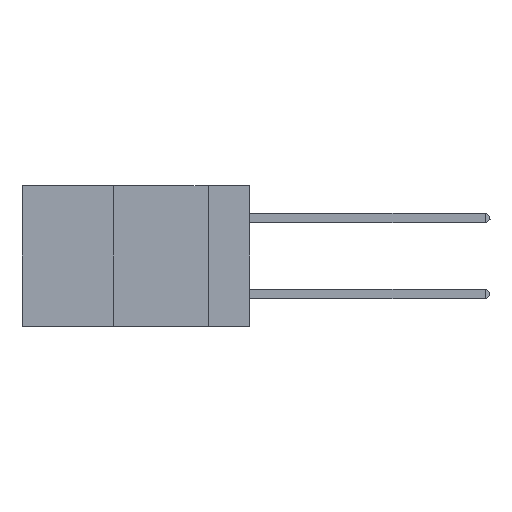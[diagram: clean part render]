
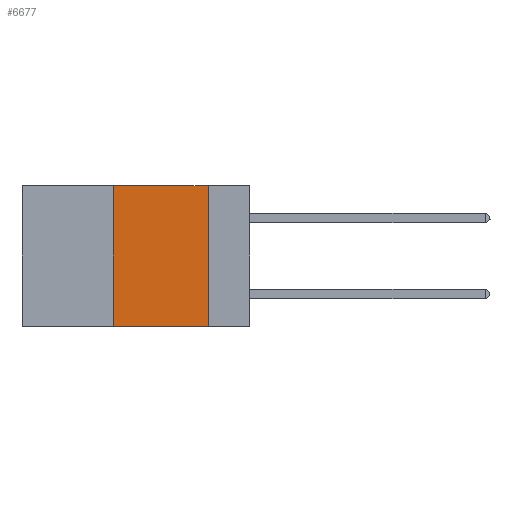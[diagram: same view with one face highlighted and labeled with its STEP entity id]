
A CAD part, left-side view. The second image highlights one B-rep face of the part: STEP entity #6677.
In plain terms, the highlighted planar face has unit normal (-1, 0, 0).
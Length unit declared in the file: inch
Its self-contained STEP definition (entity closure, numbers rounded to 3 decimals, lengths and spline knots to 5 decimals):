
#34 = LINE ( 'NONE', #2917, #3420 ) ;
#518 = DIRECTION ( 'NONE',  ( 0., 0., -1. ) ) ;
#813 = CARTESIAN_POINT ( 'NONE',  ( 0., 0.11, -0.37 ) ) ;
#999 = EDGE_CURVE ( 'NONE', #1155, #1673, #34, .T. ) ;
#1155 = VERTEX_POINT ( 'NONE', #3032 ) ;
#1369 = CARTESIAN_POINT ( 'NONE',  ( 0., 0.11, 0. ) ) ;
#1428 = VERTEX_POINT ( 'NONE', #813 ) ;
#1673 = VERTEX_POINT ( 'NONE', #4381 ) ;
#2917 = CARTESIAN_POINT ( 'NONE',  ( 0., 0.6, 0. ) ) ;
#3032 = CARTESIAN_POINT ( 'NONE',  ( 0., 0.36, 0. ) ) ;
#3420 = VECTOR ( 'NONE', #9475, 39.37008 ) ;
#4069 = EDGE_CURVE ( 'NONE', #6590, #1155, #7172, .T. ) ;
#4128 = EDGE_CURVE ( 'NONE', #1673, #1428, #5189, .T. ) ;
#4381 = CARTESIAN_POINT ( 'NONE',  ( 0., 0.11, 0. ) ) ;
#4764 = ORIENTED_EDGE ( 'NONE', *, *, #4069, .F. ) ;
#5189 = LINE ( 'NONE', #1369, #7539 ) ;
#5352 = CARTESIAN_POINT ( 'NONE',  ( 0., 0.36, -0.37 ) ) ;
#5667 = PLANE ( 'NONE',  #7354 ) ;
#6329 = DIRECTION ( 'NONE',  ( 0., 0., 1. ) ) ;
#6390 = VECTOR ( 'NONE', #10100, 39.37008 ) ;
#6590 = VERTEX_POINT ( 'NONE', #5352 ) ;
#6677 = ADVANCED_FACE ( 'NONE', ( #11259 ), #5667, .F. ) ;
#6875 = EDGE_CURVE ( 'NONE', #6590, #1428, #11846, .T. ) ;
#7172 = LINE ( 'NONE', #8108, #9311 ) ;
#7354 = AXIS2_PLACEMENT_3D ( 'NONE', #8402, #10240, #7602 ) ;
#7539 = VECTOR ( 'NONE', #518, 39.37008 ) ;
#7602 = DIRECTION ( 'NONE',  ( 0., 0., -1. ) ) ;
#8090 = EDGE_LOOP ( 'NONE', ( #11311, #10603, #4764, #8134 ) ) ;
#8108 = CARTESIAN_POINT ( 'NONE',  ( 0., 0.36, 0. ) ) ;
#8134 = ORIENTED_EDGE ( 'NONE', *, *, #6875, .T. ) ;
#8268 = CARTESIAN_POINT ( 'NONE',  ( 0., 0.6, -0.37 ) ) ;
#8402 = CARTESIAN_POINT ( 'NONE',  ( 0., 0.6, 0. ) ) ;
#9311 = VECTOR ( 'NONE', #6329, 39.37008 ) ;
#9475 = DIRECTION ( 'NONE',  ( 0., -1., 0. ) ) ;
#10100 = DIRECTION ( 'NONE',  ( 0., -1., 0. ) ) ;
#10240 = DIRECTION ( 'NONE',  ( 1., 0., 0. ) ) ;
#10603 = ORIENTED_EDGE ( 'NONE', *, *, #999, .F. ) ;
#11259 = FACE_OUTER_BOUND ( 'NONE', #8090, .T. ) ;
#11311 = ORIENTED_EDGE ( 'NONE', *, *, #4128, .F. ) ;
#11846 = LINE ( 'NONE', #8268, #6390 ) ;
